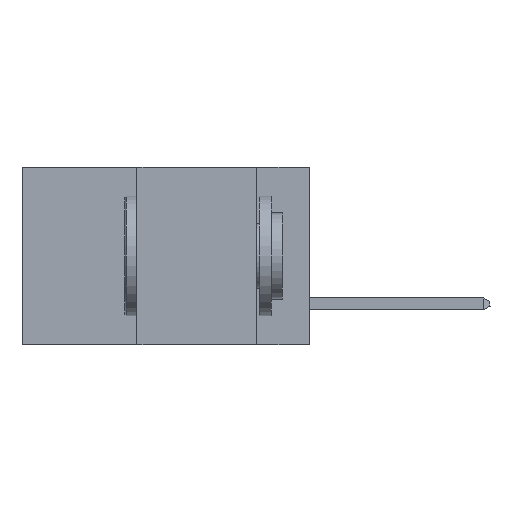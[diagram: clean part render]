
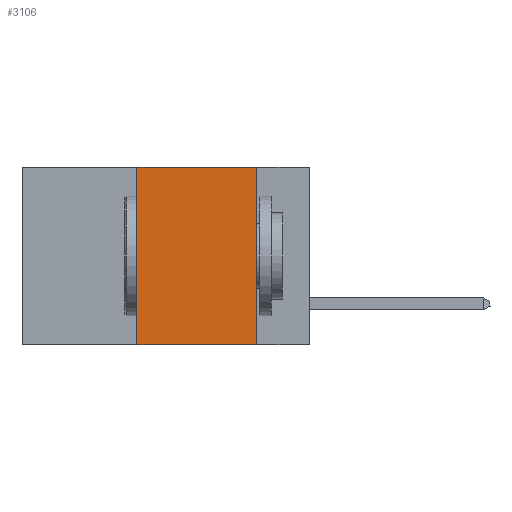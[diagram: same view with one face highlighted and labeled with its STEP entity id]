
A CAD part, left-side view. The second image highlights one B-rep face of the part: STEP entity #3106.
In plain terms, the highlighted planar face has unit normal (-1, 0, 0).
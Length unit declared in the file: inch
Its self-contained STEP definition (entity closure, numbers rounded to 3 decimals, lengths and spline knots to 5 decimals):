
#144 = VECTOR ( 'NONE', #12473, 39.37008 ) ;
#245 = DIRECTION ( 'NONE',  ( 0., -1., 0. ) ) ;
#1127 = EDGE_CURVE ( 'NONE', #9985, #9522, #11605, .T. ) ;
#1923 = ORIENTED_EDGE ( 'NONE', *, *, #1127, .F. ) ;
#1947 = DIRECTION ( 'NONE',  ( 0., 0., -1. ) ) ;
#2566 = VERTEX_POINT ( 'NONE', #11917 ) ;
#2698 = AXIS2_PLACEMENT_3D ( 'NONE', #12268, #11714, #1947 ) ;
#2915 = VECTOR ( 'NONE', #5536, 39.37008 ) ;
#3106 = ADVANCED_FACE ( 'NONE', ( #4326 ), #4457, .F. ) ;
#3593 = DIRECTION ( 'NONE',  ( 0., 0., -1. ) ) ;
#4166 = EDGE_CURVE ( 'NONE', #5144, #2566, #7547, .T. ) ;
#4326 = FACE_OUTER_BOUND ( 'NONE', #8457, .T. ) ;
#4439 = CARTESIAN_POINT ( 'NONE',  ( 0., 0.11, -0.37 ) ) ;
#4457 = PLANE ( 'NONE',  #2698 ) ;
#4896 = EDGE_CURVE ( 'NONE', #5144, #9522, #8885, .T. ) ;
#5144 = VERTEX_POINT ( 'NONE', #10194 ) ;
#5536 = DIRECTION ( 'NONE',  ( 0., 0., 1. ) ) ;
#6846 = VECTOR ( 'NONE', #245, 39.37008 ) ;
#7547 = LINE ( 'NONE', #11331, #2915 ) ;
#8029 = CARTESIAN_POINT ( 'NONE',  ( 0., 0.6, 0. ) ) ;
#8374 = ORIENTED_EDGE ( 'NONE', *, *, #4896, .T. ) ;
#8457 = EDGE_LOOP ( 'NONE', ( #1923, #9185, #9235, #8374 ) ) ;
#8563 = CARTESIAN_POINT ( 'NONE',  ( 0., 0.11, 0. ) ) ;
#8731 = VECTOR ( 'NONE', #3593, 39.37008 ) ;
#8885 = LINE ( 'NONE', #11562, #144 ) ;
#9185 = ORIENTED_EDGE ( 'NONE', *, *, #9335, .F. ) ;
#9235 = ORIENTED_EDGE ( 'NONE', *, *, #4166, .F. ) ;
#9335 = EDGE_CURVE ( 'NONE', #2566, #9985, #10793, .T. ) ;
#9522 = VERTEX_POINT ( 'NONE', #4439 ) ;
#9985 = VERTEX_POINT ( 'NONE', #8563 ) ;
#10194 = CARTESIAN_POINT ( 'NONE',  ( 0., 0.36, -0.37 ) ) ;
#10793 = LINE ( 'NONE', #8029, #6846 ) ;
#11331 = CARTESIAN_POINT ( 'NONE',  ( 0., 0.36, 0. ) ) ;
#11352 = CARTESIAN_POINT ( 'NONE',  ( 0., 0.11, 0. ) ) ;
#11562 = CARTESIAN_POINT ( 'NONE',  ( 0., 0.6, -0.37 ) ) ;
#11605 = LINE ( 'NONE', #11352, #8731 ) ;
#11714 = DIRECTION ( 'NONE',  ( 1., 0., 0. ) ) ;
#11917 = CARTESIAN_POINT ( 'NONE',  ( 0., 0.36, 0. ) ) ;
#12268 = CARTESIAN_POINT ( 'NONE',  ( 0., 0.6, 0. ) ) ;
#12473 = DIRECTION ( 'NONE',  ( 0., -1., 0. ) ) ;
